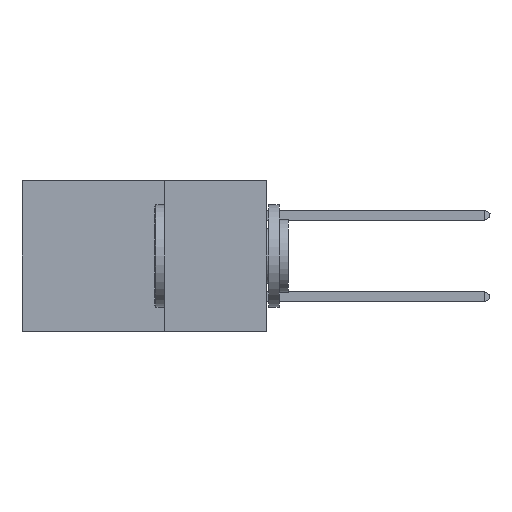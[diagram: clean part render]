
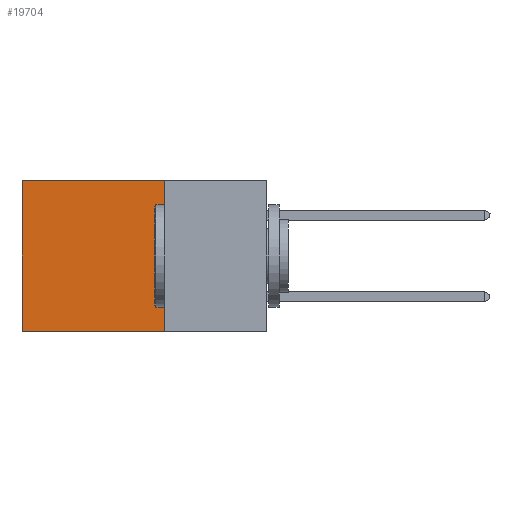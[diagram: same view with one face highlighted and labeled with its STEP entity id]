
A CAD part, left-side view. The second image highlights one B-rep face of the part: STEP entity #19704.
In plain terms, the highlighted planar face has unit normal (-1, 0, 0).
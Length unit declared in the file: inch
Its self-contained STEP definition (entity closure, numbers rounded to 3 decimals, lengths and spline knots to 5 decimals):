
#1871 = LINE ( 'NONE', #31346, #29276 ) ;
#3230 = LINE ( 'NONE', #7832, #36307 ) ;
#3402 = VERTEX_POINT ( 'NONE', #17466 ) ;
#4296 = DIRECTION ( 'NONE',  ( 0., 0., -1. ) ) ;
#4389 = ORIENTED_EDGE ( 'NONE', *, *, #8716, .F. ) ;
#4587 = DIRECTION ( 'NONE',  ( 1., 0., 0. ) ) ;
#4727 = VERTEX_POINT ( 'NONE', #29576 ) ;
#5591 = EDGE_LOOP ( 'NONE', ( #41859, #4389, #34981, #30630 ) ) ;
#5627 = FACE_OUTER_BOUND ( 'NONE', #5591, .T. ) ;
#7706 = LINE ( 'NONE', #37363, #24230 ) ;
#7832 = CARTESIAN_POINT ( 'NONE',  ( 0.2875, 0.6, 0. ) ) ;
#8716 = EDGE_CURVE ( 'NONE', #34887, #3402, #1871, .T. ) ;
#13737 = VECTOR ( 'NONE', #21928, 39.37008 ) ;
#14296 = CARTESIAN_POINT ( 'NONE',  ( 0.2875, 0.6, 0. ) ) ;
#14411 = PLANE ( 'NONE',  #29211 ) ;
#17466 = CARTESIAN_POINT ( 'NONE',  ( 0.2875, 0.6, -0.37 ) ) ;
#19677 = EDGE_CURVE ( 'NONE', #4727, #34887, #7706, .T. ) ;
#19704 = ADVANCED_FACE ( 'NONE', ( #5627 ), #14411, .F. ) ;
#21928 = DIRECTION ( 'NONE',  ( 0., 1., 0. ) ) ;
#23020 = VERTEX_POINT ( 'NONE', #14296 ) ;
#24230 = VECTOR ( 'NONE', #4296, 39.37008 ) ;
#24352 = CARTESIAN_POINT ( 'NONE',  ( 0.2875, 0.25, 0. ) ) ;
#27701 = DIRECTION ( 'NONE',  ( 0., 0., -1. ) ) ;
#28559 = CARTESIAN_POINT ( 'NONE',  ( 0.2875, 0.25, 0. ) ) ;
#29211 = AXIS2_PLACEMENT_3D ( 'NONE', #24352, #4587, #27701 ) ;
#29276 = VECTOR ( 'NONE', #34651, 39.37008 ) ;
#29576 = CARTESIAN_POINT ( 'NONE',  ( 0.2875, 0.25, 0. ) ) ;
#30630 = ORIENTED_EDGE ( 'NONE', *, *, #34311, .T. ) ;
#31346 = CARTESIAN_POINT ( 'NONE',  ( 0.2875, 0.25, -0.37 ) ) ;
#34134 = DIRECTION ( 'NONE',  ( 0., 0., -1. ) ) ;
#34311 = EDGE_CURVE ( 'NONE', #4727, #23020, #39019, .T. ) ;
#34651 = DIRECTION ( 'NONE',  ( 0., 1., 0. ) ) ;
#34887 = VERTEX_POINT ( 'NONE', #41219 ) ;
#34981 = ORIENTED_EDGE ( 'NONE', *, *, #19677, .F. ) ;
#36307 = VECTOR ( 'NONE', #34134, 39.37008 ) ;
#37363 = CARTESIAN_POINT ( 'NONE',  ( 0.2875, 0.25, 0. ) ) ;
#39019 = LINE ( 'NONE', #28559, #13737 ) ;
#41219 = CARTESIAN_POINT ( 'NONE',  ( 0.2875, 0.25, -0.37 ) ) ;
#41286 = EDGE_CURVE ( 'NONE', #23020, #3402, #3230, .T. ) ;
#41859 = ORIENTED_EDGE ( 'NONE', *, *, #41286, .T. ) ;
